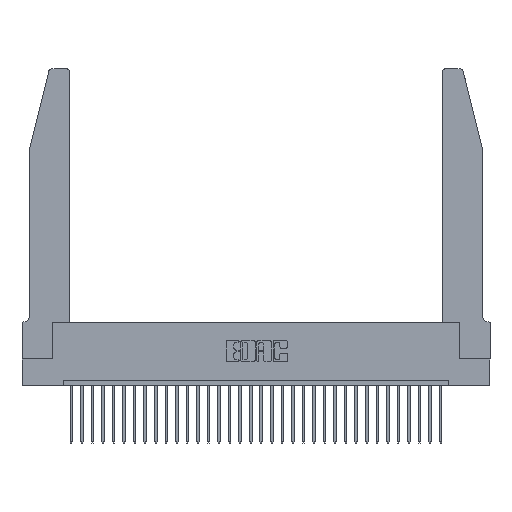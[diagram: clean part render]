
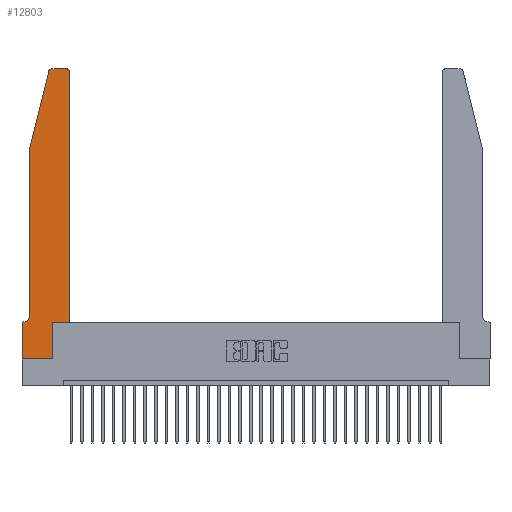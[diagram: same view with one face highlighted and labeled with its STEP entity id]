
A CAD part, top view. The second image highlights one B-rep face of the part: STEP entity #12803.
In plain terms, the highlighted planar face has unit normal (0, 0, 1).
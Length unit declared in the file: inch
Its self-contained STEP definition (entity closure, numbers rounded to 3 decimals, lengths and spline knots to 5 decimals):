
#791 = LINE ( 'NONE', #17528, #20116 ) ;
#1176 = VECTOR ( 'NONE', #20260, 39.37008 ) ;
#1482 = CIRCLE ( 'NONE', #14663, 0.03 ) ;
#1887 = ORIENTED_EDGE ( 'NONE', *, *, #30224, .T. ) ;
#1955 = CARTESIAN_POINT ( 'NONE',  ( 0.4505, 2.72, 0.37 ) ) ;
#2038 = CARTESIAN_POINT ( 'NONE',  ( 0.0755, 0.42, 0.37 ) ) ;
#2509 = CARTESIAN_POINT ( 'NONE',  ( 0., 0.35, 0.37 ) ) ;
#2518 = VERTEX_POINT ( 'NONE', #2038 ) ;
#2988 = CARTESIAN_POINT ( 'NONE',  ( 0.0055, 0.35, 0.37 ) ) ;
#3202 = VERTEX_POINT ( 'NONE', #2509 ) ;
#3358 = VERTEX_POINT ( 'NONE', #22985 ) ;
#3410 = EDGE_CURVE ( 'NONE', #3358, #28101, #20624, .T. ) ;
#3765 = DIRECTION ( 'NONE',  ( -1., 0., 0. ) ) ;
#4691 = DIRECTION ( 'NONE',  ( 0., 0., -1. ) ) ;
#4797 = ORIENTED_EDGE ( 'NONE', *, *, #18227, .T. ) ;
#5060 = VERTEX_POINT ( 'NONE', #2988 ) ;
#5282 = CARTESIAN_POINT ( 'NONE',  ( 0., 0., 0.37 ) ) ;
#5997 = AXIS2_PLACEMENT_3D ( 'NONE', #11702, #29568, #19480 ) ;
#6133 = ORIENTED_EDGE ( 'NONE', *, *, #32127, .T. ) ;
#6350 = CARTESIAN_POINT ( 'NONE',  ( 0.284, 2.72, 0.37 ) ) ;
#6428 = EDGE_CURVE ( 'NONE', #9236, #22660, #13266, .T. ) ;
#6504 = VERTEX_POINT ( 'NONE', #1955 ) ;
#6505 = LINE ( 'NONE', #5282, #14814 ) ;
#6622 = ORIENTED_EDGE ( 'NONE', *, *, #8502, .T. ) ;
#6654 = DIRECTION ( 'NONE',  ( -0.239, -0.971, 0. ) ) ;
#7213 = VERTEX_POINT ( 'NONE', #25248 ) ;
#8310 = CARTESIAN_POINT ( 'NONE',  ( 0.2605, 2.75, 0.37 ) ) ;
#8502 = EDGE_CURVE ( 'NONE', #6504, #3358, #30922, .T. ) ;
#8684 = ORIENTED_EDGE ( 'NONE', *, *, #9176, .T. ) ;
#8812 = VECTOR ( 'NONE', #20994, 39.37008 ) ;
#8878 = DIRECTION ( 'NONE',  ( 0., 0., 1. ) ) ;
#9176 = EDGE_CURVE ( 'NONE', #7213, #14226, #791, .T. ) ;
#9236 = VERTEX_POINT ( 'NONE', #18292 ) ;
#9517 = CARTESIAN_POINT ( 'NONE',  ( 0.0755, 2., 0.37 ) ) ;
#9933 = VECTOR ( 'NONE', #18285, 39.37008 ) ;
#9945 = EDGE_CURVE ( 'NONE', #5060, #3202, #29166, .T. ) ;
#10832 = CARTESIAN_POINT ( 'NONE',  ( 0.2865, 0., 0.37 ) ) ;
#11702 = CARTESIAN_POINT ( 'NONE',  ( 0.4205, 2.72, 0.37 ) ) ;
#12078 = CARTESIAN_POINT ( 'NONE',  ( 0.0755, 2., 0.37 ) ) ;
#12093 = VECTOR ( 'NONE', #6654, 39.37008 ) ;
#12367 = AXIS2_PLACEMENT_3D ( 'NONE', #19822, #4691, #22956 ) ;
#12722 = EDGE_CURVE ( 'NONE', #14226, #25151, #30525, .T. ) ;
#12803 = ADVANCED_FACE ( 'NONE', ( #13933 ), #13891, .T. ) ;
#13266 = LINE ( 'NONE', #9517, #12093 ) ;
#13891 = PLANE ( 'NONE',  #30389 ) ;
#13933 = FACE_OUTER_BOUND ( 'NONE', #17576, .T. ) ;
#14224 = CARTESIAN_POINT ( 'NONE',  ( 0., 0.35, 0.37 ) ) ;
#14226 = VERTEX_POINT ( 'NONE', #10832 ) ;
#14274 = CARTESIAN_POINT ( 'NONE',  ( 0.0755, 2., 0.37 ) ) ;
#14330 = DIRECTION ( 'NONE',  ( 1., 0., 0. ) ) ;
#14547 = LINE ( 'NONE', #14274, #27953 ) ;
#14663 = AXIS2_PLACEMENT_3D ( 'NONE', #6350, #8878, #22127 ) ;
#14814 = VECTOR ( 'NONE', #22921, 39.37008 ) ;
#14897 = ORIENTED_EDGE ( 'NONE', *, *, #3410, .T. ) ;
#15037 = ORIENTED_EDGE ( 'NONE', *, *, #19170, .T. ) ;
#16531 = ORIENTED_EDGE ( 'NONE', *, *, #9945, .T. ) ;
#17528 = CARTESIAN_POINT ( 'NONE',  ( 0., 0., 0.37 ) ) ;
#17576 = EDGE_LOOP ( 'NONE', ( #14897, #4797, #27402, #28274, #1887, #16531, #15037, #8684, #21487, #26686, #6133, #6622 ) ) ;
#18227 = EDGE_CURVE ( 'NONE', #28101, #9236, #1482, .T. ) ;
#18285 = DIRECTION ( 'NONE',  ( -1., 0., 0. ) ) ;
#18292 = CARTESIAN_POINT ( 'NONE',  ( 0.25487, 2.72718, 0.37 ) ) ;
#19099 = LINE ( 'NONE', #31729, #24942 ) ;
#19170 = EDGE_CURVE ( 'NONE', #3202, #7213, #6505, .T. ) ;
#19480 = DIRECTION ( 'NONE',  ( 1., 0., 0. ) ) ;
#19546 = DIRECTION ( 'NONE',  ( 1., 0., 0. ) ) ;
#19822 = CARTESIAN_POINT ( 'NONE',  ( 0.0055, 0.42, 0.37 ) ) ;
#20116 = VECTOR ( 'NONE', #25083, 39.37008 ) ;
#20260 = DIRECTION ( 'NONE',  ( 0., 1., 0. ) ) ;
#20423 = VERTEX_POINT ( 'NONE', #27362 ) ;
#20446 = EDGE_CURVE ( 'NONE', #25151, #20423, #19099, .T. ) ;
#20624 = LINE ( 'NONE', #8310, #9933 ) ;
#20994 = DIRECTION ( 'NONE',  ( 0., 1., 0. ) ) ;
#21487 = ORIENTED_EDGE ( 'NONE', *, *, #12722, .T. ) ;
#21683 = VECTOR ( 'NONE', #3765, 39.37008 ) ;
#22127 = DIRECTION ( 'NONE',  ( 1., 0., 0. ) ) ;
#22660 = VERTEX_POINT ( 'NONE', #12078 ) ;
#22921 = DIRECTION ( 'NONE',  ( 0., -1., 0. ) ) ;
#22956 = DIRECTION ( 'NONE',  ( -1., 0., 0. ) ) ;
#22985 = CARTESIAN_POINT ( 'NONE',  ( 0.4205, 2.75, 0.37 ) ) ;
#24211 = CARTESIAN_POINT ( 'NONE',  ( 0.0755, 0.35, 0.37 ) ) ;
#24370 = DIRECTION ( 'NONE',  ( 0., 0., 1. ) ) ;
#24942 = VECTOR ( 'NONE', #19546, 39.37008 ) ;
#25083 = DIRECTION ( 'NONE',  ( 1., 0., 0. ) ) ;
#25151 = VERTEX_POINT ( 'NONE', #31451 ) ;
#25248 = CARTESIAN_POINT ( 'NONE',  ( 0., 0., 0.37 ) ) ;
#26480 = CIRCLE ( 'NONE', #12367, 0.07 ) ;
#26686 = ORIENTED_EDGE ( 'NONE', *, *, #20446, .T. ) ;
#27362 = CARTESIAN_POINT ( 'NONE',  ( 0.4505, 0.35, 0.37 ) ) ;
#27402 = ORIENTED_EDGE ( 'NONE', *, *, #6428, .T. ) ;
#27953 = VECTOR ( 'NONE', #29508, 39.37008 ) ;
#28101 = VERTEX_POINT ( 'NONE', #30822 ) ;
#28274 = ORIENTED_EDGE ( 'NONE', *, *, #32090, .T. ) ;
#28751 = LINE ( 'NONE', #29725, #1176 ) ;
#29166 = LINE ( 'NONE', #24211, #21683 ) ;
#29508 = DIRECTION ( 'NONE',  ( 0., -1., 0. ) ) ;
#29568 = DIRECTION ( 'NONE',  ( 0., 0., 1. ) ) ;
#29725 = CARTESIAN_POINT ( 'NONE',  ( 0.4505, 0.35, 0.37 ) ) ;
#30224 = EDGE_CURVE ( 'NONE', #2518, #5060, #26480, .T. ) ;
#30389 = AXIS2_PLACEMENT_3D ( 'NONE', #14224, #24370, #14330 ) ;
#30525 = LINE ( 'NONE', #31025, #8812 ) ;
#30822 = CARTESIAN_POINT ( 'NONE',  ( 0.284, 2.75, 0.37 ) ) ;
#30922 = CIRCLE ( 'NONE', #5997, 0.03 ) ;
#31025 = CARTESIAN_POINT ( 'NONE',  ( 0.2865, 0.35, 0.37 ) ) ;
#31451 = CARTESIAN_POINT ( 'NONE',  ( 0.2865, 0.35, 0.37 ) ) ;
#31729 = CARTESIAN_POINT ( 'NONE',  ( 0.4505, 0.35, 0.37 ) ) ;
#32090 = EDGE_CURVE ( 'NONE', #22660, #2518, #14547, .T. ) ;
#32127 = EDGE_CURVE ( 'NONE', #20423, #6504, #28751, .T. ) ;
